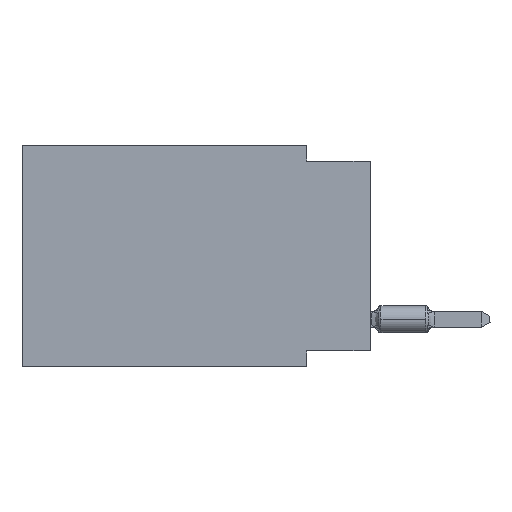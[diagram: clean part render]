
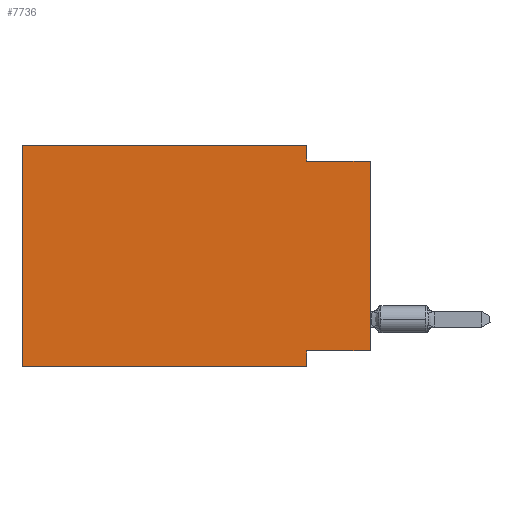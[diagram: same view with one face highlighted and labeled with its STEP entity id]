
A CAD part, left-side view. The second image highlights one B-rep face of the part: STEP entity #7736.
In plain terms, the highlighted planar face has unit normal (-1, 0, 0).
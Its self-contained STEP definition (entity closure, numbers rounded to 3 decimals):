
#25 = DIRECTION ( 'NONE',  ( 0., 0., 1. ) ) ;
#429 = VECTOR ( 'NONE', #51749, 1000. ) ;
#639 = VECTOR ( 'NONE', #6487, 1000. ) ;
#1632 = EDGE_CURVE ( 'NONE', #30489, #34293, #25143, .T. ) ;
#1667 = VERTEX_POINT ( 'NONE', #29267 ) ;
#3110 = CARTESIAN_POINT ( 'NONE',  ( 0., 13.97, 0. ) ) ;
#5524 = VERTEX_POINT ( 'NONE', #36352 ) ;
#6487 = DIRECTION ( 'NONE',  ( 0., 0., -1. ) ) ;
#6552 = EDGE_LOOP ( 'NONE', ( #30189, #11643, #6918, #26693, #15636, #32025, #43236, #24361 ) ) ;
#6918 = ORIENTED_EDGE ( 'NONE', *, *, #21214, .F. ) ;
#7528 = CARTESIAN_POINT ( 'NONE',  ( 0., 13.97, 0. ) ) ;
#7736 = ADVANCED_FACE ( 'NONE', ( #33748 ), #42294, .F. ) ;
#8909 = CARTESIAN_POINT ( 'NONE',  ( 0., 0., 0. ) ) ;
#9962 = DIRECTION ( 'NONE',  ( 0., 0., -1. ) ) ;
#10551 = CARTESIAN_POINT ( 'NONE',  ( 0., 13.97, 0. ) ) ;
#11203 = CARTESIAN_POINT ( 'NONE',  ( 0., 2.54, -8.89 ) ) ;
#11313 = DIRECTION ( 'NONE',  ( 0., -1., 0. ) ) ;
#11643 = ORIENTED_EDGE ( 'NONE', *, *, #16443, .F. ) ;
#12254 = VECTOR ( 'NONE', #11313, 1000. ) ;
#12925 = AXIS2_PLACEMENT_3D ( 'NONE', #7528, #33462, #29333 ) ;
#13515 = LINE ( 'NONE', #41198, #44635 ) ;
#15636 = ORIENTED_EDGE ( 'NONE', *, *, #48383, .F. ) ;
#16443 = EDGE_CURVE ( 'NONE', #5524, #53425, #19875, .T. ) ;
#16586 = VECTOR ( 'NONE', #25, 1000. ) ;
#18066 = VERTEX_POINT ( 'NONE', #53469 ) ;
#19389 = CARTESIAN_POINT ( 'NONE',  ( 0., 13.97, -8.89 ) ) ;
#19414 = CARTESIAN_POINT ( 'NONE',  ( 0., 0., -8.255 ) ) ;
#19875 = LINE ( 'NONE', #20156, #12254 ) ;
#20156 = CARTESIAN_POINT ( 'NONE',  ( 0., 0., -0.635 ) ) ;
#21214 = EDGE_CURVE ( 'NONE', #34293, #5524, #13515, .T. ) ;
#21458 = EDGE_CURVE ( 'NONE', #1667, #58167, #38227, .T. ) ;
#21951 = VECTOR ( 'NONE', #38106, 1000. ) ;
#22453 = CARTESIAN_POINT ( 'NONE',  ( 0., 2.54, -8.89 ) ) ;
#24361 = ORIENTED_EDGE ( 'NONE', *, *, #35885, .F. ) ;
#24404 = LINE ( 'NONE', #10551, #52173 ) ;
#25143 = LINE ( 'NONE', #28677, #21951 ) ;
#26693 = ORIENTED_EDGE ( 'NONE', *, *, #1632, .F. ) ;
#28677 = CARTESIAN_POINT ( 'NONE',  ( 0., 13.97, 0. ) ) ;
#29267 = CARTESIAN_POINT ( 'NONE',  ( 0., 13.97, -8.89 ) ) ;
#29333 = DIRECTION ( 'NONE',  ( 0., 0., -1. ) ) ;
#30189 = ORIENTED_EDGE ( 'NONE', *, *, #40613, .T. ) ;
#30489 = VERTEX_POINT ( 'NONE', #3110 ) ;
#31850 = VECTOR ( 'NONE', #32953, 1000. ) ;
#32025 = ORIENTED_EDGE ( 'NONE', *, *, #21458, .T. ) ;
#32953 = DIRECTION ( 'NONE',  ( 0., 1., 0. ) ) ;
#33462 = DIRECTION ( 'NONE',  ( 1., 0., 0. ) ) ;
#33748 = FACE_OUTER_BOUND ( 'NONE', #6552, .T. ) ;
#34293 = VERTEX_POINT ( 'NONE', #35366 ) ;
#35366 = CARTESIAN_POINT ( 'NONE',  ( 0., 2.54, 0. ) ) ;
#35885 = EDGE_CURVE ( 'NONE', #52171, #18066, #45348, .T. ) ;
#36352 = CARTESIAN_POINT ( 'NONE',  ( 0., 2.54, -0.635 ) ) ;
#38106 = DIRECTION ( 'NONE',  ( 0., -1., 0. ) ) ;
#38227 = LINE ( 'NONE', #19389, #429 ) ;
#40613 = EDGE_CURVE ( 'NONE', #52171, #53425, #45709, .T. ) ;
#41198 = CARTESIAN_POINT ( 'NONE',  ( 0., 2.54, 0. ) ) ;
#41562 = CARTESIAN_POINT ( 'NONE',  ( 0., 0., -8.255 ) ) ;
#41694 = EDGE_CURVE ( 'NONE', #18066, #58167, #51548, .T. ) ;
#42294 = PLANE ( 'NONE',  #12925 ) ;
#43236 = ORIENTED_EDGE ( 'NONE', *, *, #41694, .F. ) ;
#44635 = VECTOR ( 'NONE', #9962, 1000. ) ;
#45348 = LINE ( 'NONE', #19414, #31850 ) ;
#45709 = LINE ( 'NONE', #8909, #16586 ) ;
#48383 = EDGE_CURVE ( 'NONE', #1667, #30489, #24404, .T. ) ;
#50115 = CARTESIAN_POINT ( 'NONE',  ( 0., 0., -0.635 ) ) ;
#51548 = LINE ( 'NONE', #11203, #639 ) ;
#51749 = DIRECTION ( 'NONE',  ( 0., -1., 0. ) ) ;
#52171 = VERTEX_POINT ( 'NONE', #41562 ) ;
#52173 = VECTOR ( 'NONE', #55610, 1000. ) ;
#53425 = VERTEX_POINT ( 'NONE', #50115 ) ;
#53469 = CARTESIAN_POINT ( 'NONE',  ( 0., 2.54, -8.255 ) ) ;
#55610 = DIRECTION ( 'NONE',  ( 0., 0., 1. ) ) ;
#58167 = VERTEX_POINT ( 'NONE', #22453 ) ;
